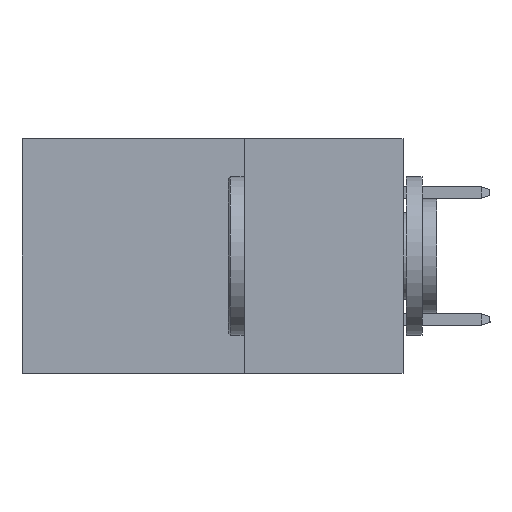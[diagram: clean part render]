
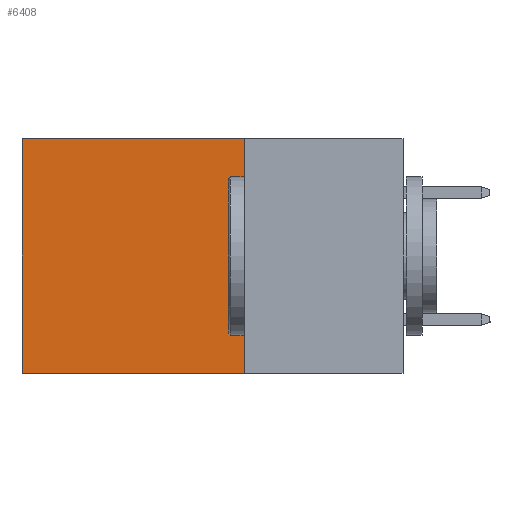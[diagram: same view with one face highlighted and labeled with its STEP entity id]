
A CAD part, left-side view. The second image highlights one B-rep face of the part: STEP entity #6408.
In plain terms, the highlighted planar face has unit normal (-1, 0, 0).
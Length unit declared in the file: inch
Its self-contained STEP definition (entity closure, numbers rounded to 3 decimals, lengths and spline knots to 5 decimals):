
#60 = CARTESIAN_POINT ( 'NONE',  ( 0.2875, 0.25, 0. ) ) ;
#125 = VERTEX_POINT ( 'NONE', #11369 ) ;
#938 = CARTESIAN_POINT ( 'NONE',  ( 0.2875, 0.25, 0. ) ) ;
#2198 = FACE_OUTER_BOUND ( 'NONE', #3025, .T. ) ;
#2686 = ORIENTED_EDGE ( 'NONE', *, *, #8823, .F. ) ;
#2948 = CARTESIAN_POINT ( 'NONE',  ( 0.2875, 0.25, 0. ) ) ;
#3025 = EDGE_LOOP ( 'NONE', ( #3906, #19434, #2686, #11306 ) ) ;
#3906 = ORIENTED_EDGE ( 'NONE', *, *, #7812, .T. ) ;
#4015 = CARTESIAN_POINT ( 'NONE',  ( 0.2875, 0.25, 0. ) ) ;
#5568 = PLANE ( 'NONE',  #19180 ) ;
#6408 = ADVANCED_FACE ( 'NONE', ( #2198 ), #5568, .F. ) ;
#6759 = LINE ( 'NONE', #7173, #12446 ) ;
#7173 = CARTESIAN_POINT ( 'NONE',  ( 0.2875, 0.6, 0. ) ) ;
#7812 = EDGE_CURVE ( 'NONE', #19195, #125, #6759, .T. ) ;
#7825 = LINE ( 'NONE', #18996, #12733 ) ;
#8823 = EDGE_CURVE ( 'NONE', #18967, #8963, #20224, .T. ) ;
#8963 = VERTEX_POINT ( 'NONE', #11024 ) ;
#10292 = EDGE_CURVE ( 'NONE', #8963, #125, #7825, .T. ) ;
#11024 = CARTESIAN_POINT ( 'NONE',  ( 0.2875, 0.25, -0.37 ) ) ;
#11048 = DIRECTION ( 'NONE',  ( 0., 1., 0. ) ) ;
#11306 = ORIENTED_EDGE ( 'NONE', *, *, #12696, .T. ) ;
#11369 = CARTESIAN_POINT ( 'NONE',  ( 0.2875, 0.6, -0.37 ) ) ;
#11933 = DIRECTION ( 'NONE',  ( 0., 0., -1. ) ) ;
#11948 = VECTOR ( 'NONE', #20247, 39.37008 ) ;
#12446 = VECTOR ( 'NONE', #14897, 39.37008 ) ;
#12696 = EDGE_CURVE ( 'NONE', #18967, #19195, #13742, .T. ) ;
#12733 = VECTOR ( 'NONE', #11048, 39.37008 ) ;
#13607 = DIRECTION ( 'NONE',  ( 1., 0., 0. ) ) ;
#13742 = LINE ( 'NONE', #4015, #11948 ) ;
#14057 = VECTOR ( 'NONE', #16957, 39.37008 ) ;
#14897 = DIRECTION ( 'NONE',  ( 0., 0., -1. ) ) ;
#16957 = DIRECTION ( 'NONE',  ( 0., 0., -1. ) ) ;
#18363 = CARTESIAN_POINT ( 'NONE',  ( 0.2875, 0.6, 0. ) ) ;
#18967 = VERTEX_POINT ( 'NONE', #60 ) ;
#18996 = CARTESIAN_POINT ( 'NONE',  ( 0.2875, 0.25, -0.37 ) ) ;
#19180 = AXIS2_PLACEMENT_3D ( 'NONE', #938, #13607, #11933 ) ;
#19195 = VERTEX_POINT ( 'NONE', #18363 ) ;
#19434 = ORIENTED_EDGE ( 'NONE', *, *, #10292, .F. ) ;
#20224 = LINE ( 'NONE', #2948, #14057 ) ;
#20247 = DIRECTION ( 'NONE',  ( 0., 1., 0. ) ) ;
